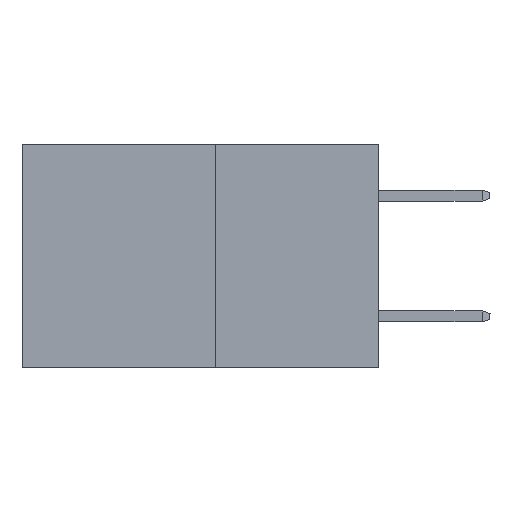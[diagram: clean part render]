
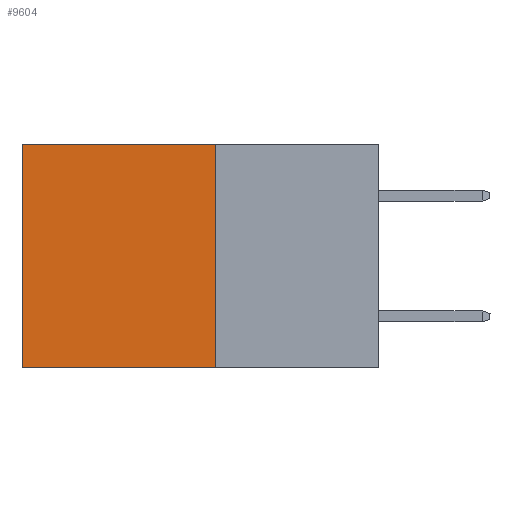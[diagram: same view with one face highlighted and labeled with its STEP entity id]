
A CAD part, left-side view. The second image highlights one B-rep face of the part: STEP entity #9604.
In plain terms, the highlighted planar face has unit normal (-1, 0, 0).
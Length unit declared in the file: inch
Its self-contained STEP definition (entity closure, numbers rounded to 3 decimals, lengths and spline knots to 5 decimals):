
#297 = CARTESIAN_POINT ( 'NONE',  ( 0.277, 0.27, -0.37 ) ) ;
#393 = AXIS2_PLACEMENT_3D ( 'NONE', #15900, #20903, #5849 ) ;
#1653 = CARTESIAN_POINT ( 'NONE',  ( 0.277, 0.27, 0. ) ) ;
#2812 = VECTOR ( 'NONE', #20437, 39.37008 ) ;
#3290 = LINE ( 'NONE', #26703, #28284 ) ;
#4420 = LINE ( 'NONE', #1653, #29382 ) ;
#5849 = DIRECTION ( 'NONE',  ( 0., 0., -1. ) ) ;
#6322 = VECTOR ( 'NONE', #26427, 39.37008 ) ;
#8291 = PLANE ( 'NONE',  #393 ) ;
#9110 = CARTESIAN_POINT ( 'NONE',  ( 0.277, 0.59, -0.37 ) ) ;
#9604 = ADVANCED_FACE ( 'NONE', ( #20833 ), #8291, .F. ) ;
#11606 = CARTESIAN_POINT ( 'NONE',  ( 0.277, 0.59, -0.37 ) ) ;
#12907 = ORIENTED_EDGE ( 'NONE', *, *, #14760, .T. ) ;
#14260 = DIRECTION ( 'NONE',  ( 0., 1., 0. ) ) ;
#14760 = EDGE_CURVE ( 'NONE', #31798, #26748, #4420, .T. ) ;
#15531 = ORIENTED_EDGE ( 'NONE', *, *, #20178, .F. ) ;
#15831 = EDGE_LOOP ( 'NONE', ( #16441, #18602, #15531, #12907 ) ) ;
#15900 = CARTESIAN_POINT ( 'NONE',  ( 0.277, 0.27, -0.37 ) ) ;
#16441 = ORIENTED_EDGE ( 'NONE', *, *, #21159, .T. ) ;
#16628 = CARTESIAN_POINT ( 'NONE',  ( 0.277, 0.27, -0.37 ) ) ;
#18602 = ORIENTED_EDGE ( 'NONE', *, *, #21928, .F. ) ;
#18866 = CARTESIAN_POINT ( 'NONE',  ( 0.277, 0.27, 0. ) ) ;
#19692 = LINE ( 'NONE', #11606, #6322 ) ;
#20178 = EDGE_CURVE ( 'NONE', #31798, #27271, #29378, .T. ) ;
#20437 = DIRECTION ( 'NONE',  ( 0., 0., -1. ) ) ;
#20833 = FACE_OUTER_BOUND ( 'NONE', #15831, .T. ) ;
#20903 = DIRECTION ( 'NONE',  ( 1., 0., 0. ) ) ;
#21159 = EDGE_CURVE ( 'NONE', #26748, #21185, #19692, .T. ) ;
#21185 = VERTEX_POINT ( 'NONE', #9110 ) ;
#21928 = EDGE_CURVE ( 'NONE', #27271, #21185, #3290, .T. ) ;
#26427 = DIRECTION ( 'NONE',  ( 0., 0., -1. ) ) ;
#26703 = CARTESIAN_POINT ( 'NONE',  ( 0.277, 0.27, -0.37 ) ) ;
#26748 = VERTEX_POINT ( 'NONE', #26912 ) ;
#26912 = CARTESIAN_POINT ( 'NONE',  ( 0.277, 0.59, 0. ) ) ;
#27271 = VERTEX_POINT ( 'NONE', #16628 ) ;
#28284 = VECTOR ( 'NONE', #29166, 39.37008 ) ;
#29166 = DIRECTION ( 'NONE',  ( 0., 1., 0. ) ) ;
#29378 = LINE ( 'NONE', #297, #2812 ) ;
#29382 = VECTOR ( 'NONE', #14260, 39.37008 ) ;
#31798 = VERTEX_POINT ( 'NONE', #18866 ) ;
